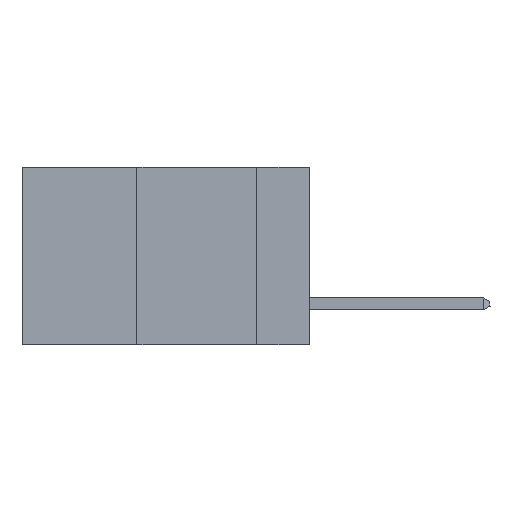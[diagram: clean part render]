
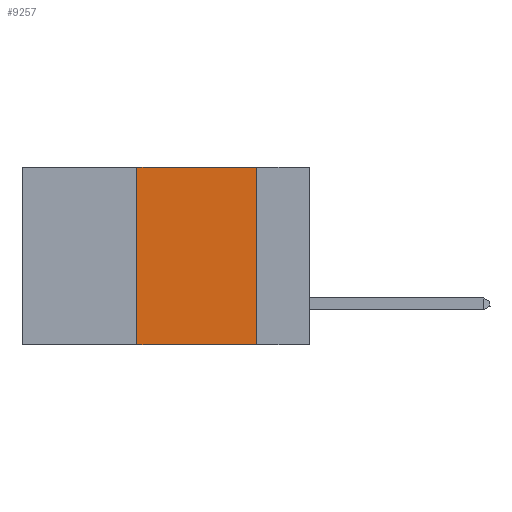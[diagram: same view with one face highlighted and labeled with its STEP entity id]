
A CAD part, left-side view. The second image highlights one B-rep face of the part: STEP entity #9257.
In plain terms, the highlighted planar face has unit normal (-1, 0, 0).
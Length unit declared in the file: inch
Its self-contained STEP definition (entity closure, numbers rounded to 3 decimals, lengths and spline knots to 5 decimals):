
#114 = DIRECTION ( 'NONE',  ( 1., 0., 0. ) ) ;
#487 = ORIENTED_EDGE ( 'NONE', *, *, #13759, .F. ) ;
#853 = CARTESIAN_POINT ( 'NONE',  ( 0., 0.11, 0. ) ) ;
#1299 = VERTEX_POINT ( 'NONE', #853 ) ;
#3371 = ORIENTED_EDGE ( 'NONE', *, *, #24425, .T. ) ;
#3496 = CARTESIAN_POINT ( 'NONE',  ( 0., 0.11, 0. ) ) ;
#3548 = AXIS2_PLACEMENT_3D ( 'NONE', #20066, #114, #8158 ) ;
#3982 = VECTOR ( 'NONE', #17492, 39.37008 ) ;
#4005 = EDGE_LOOP ( 'NONE', ( #487, #13945, #20252, #3371 ) ) ;
#6236 = PLANE ( 'NONE',  #3548 ) ;
#8158 = DIRECTION ( 'NONE',  ( 0., 0., -1. ) ) ;
#8344 = LINE ( 'NONE', #3496, #18848 ) ;
#8630 = CARTESIAN_POINT ( 'NONE',  ( 0., 0.36, 0. ) ) ;
#8826 = VERTEX_POINT ( 'NONE', #25145 ) ;
#9058 = CARTESIAN_POINT ( 'NONE',  ( 0., 0.6, 0. ) ) ;
#9257 = ADVANCED_FACE ( 'NONE', ( #24438 ), #6236, .F. ) ;
#10228 = CARTESIAN_POINT ( 'NONE',  ( 0., 0.36, 0. ) ) ;
#11594 = LINE ( 'NONE', #9058, #18450 ) ;
#13011 = VECTOR ( 'NONE', #18026, 39.37008 ) ;
#13759 = EDGE_CURVE ( 'NONE', #1299, #24709, #8344, .T. ) ;
#13945 = ORIENTED_EDGE ( 'NONE', *, *, #20276, .F. ) ;
#15488 = CARTESIAN_POINT ( 'NONE',  ( 0., 0.6, -0.37 ) ) ;
#17055 = DIRECTION ( 'NONE',  ( 0., 0., -1. ) ) ;
#17492 = DIRECTION ( 'NONE',  ( 0., -1., 0. ) ) ;
#18026 = DIRECTION ( 'NONE',  ( 0., 0., 1. ) ) ;
#18251 = LINE ( 'NONE', #15488, #3982 ) ;
#18295 = LINE ( 'NONE', #10228, #13011 ) ;
#18450 = VECTOR ( 'NONE', #20979, 39.37008 ) ;
#18848 = VECTOR ( 'NONE', #17055, 39.37008 ) ;
#20066 = CARTESIAN_POINT ( 'NONE',  ( 0., 0.6, 0. ) ) ;
#20252 = ORIENTED_EDGE ( 'NONE', *, *, #24894, .F. ) ;
#20276 = EDGE_CURVE ( 'NONE', #21378, #1299, #11594, .T. ) ;
#20979 = DIRECTION ( 'NONE',  ( 0., -1., 0. ) ) ;
#21378 = VERTEX_POINT ( 'NONE', #8630 ) ;
#24288 = CARTESIAN_POINT ( 'NONE',  ( 0., 0.11, -0.37 ) ) ;
#24425 = EDGE_CURVE ( 'NONE', #8826, #24709, #18251, .T. ) ;
#24438 = FACE_OUTER_BOUND ( 'NONE', #4005, .T. ) ;
#24709 = VERTEX_POINT ( 'NONE', #24288 ) ;
#24894 = EDGE_CURVE ( 'NONE', #8826, #21378, #18295, .T. ) ;
#25145 = CARTESIAN_POINT ( 'NONE',  ( 0., 0.36, -0.37 ) ) ;
